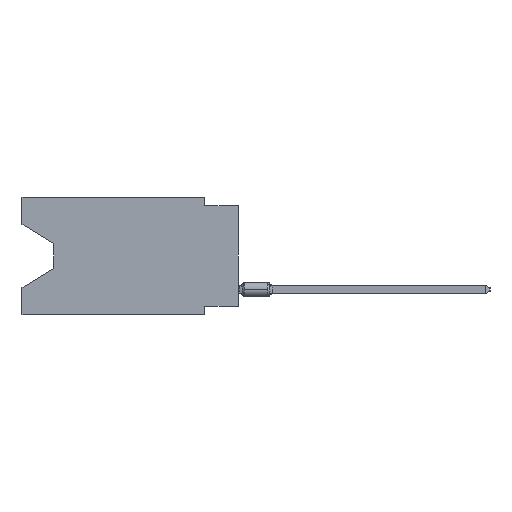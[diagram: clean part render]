
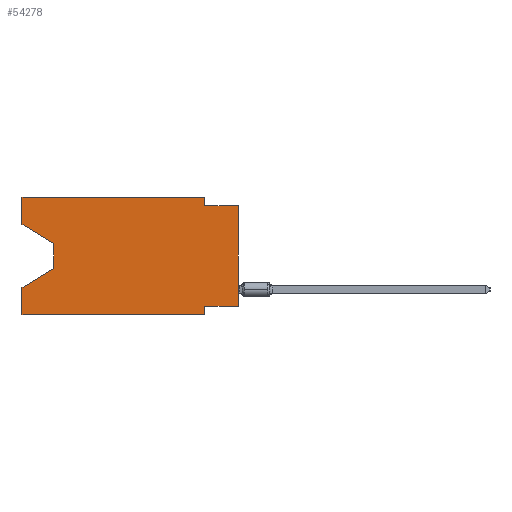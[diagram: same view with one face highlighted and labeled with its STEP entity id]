
A CAD part, left-side view. The second image highlights one B-rep face of the part: STEP entity #54278.
In plain terms, the highlighted planar face has unit normal (-1, 0, 0).
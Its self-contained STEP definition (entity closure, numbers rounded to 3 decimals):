
#98 = VERTEX_POINT ( 'NONE', #68388 ) ;
#173 = CARTESIAN_POINT ( 'NONE',  ( 0., 16.383, -2.038 ) ) ;
#647 = LINE ( 'NONE', #6383, #62513 ) ;
#803 = VERTEX_POINT ( 'NONE', #11691 ) ;
#1024 = CARTESIAN_POINT ( 'NONE',  ( 0., 2.54, 0. ) ) ;
#2046 = CARTESIAN_POINT ( 'NONE',  ( 0., 0., -0.635 ) ) ;
#2863 = CARTESIAN_POINT ( 'NONE',  ( 0., 0., -8.255 ) ) ;
#4618 = VECTOR ( 'NONE', #35750, 1000. ) ;
#4832 = ORIENTED_EDGE ( 'NONE', *, *, #60433, .F. ) ;
#4844 = DIRECTION ( 'NONE',  ( 1., 0., 0. ) ) ;
#5903 = ORIENTED_EDGE ( 'NONE', *, *, #38553, .F. ) ;
#6383 = CARTESIAN_POINT ( 'NONE',  ( 0., 2.54, -8.89 ) ) ;
#6622 = VERTEX_POINT ( 'NONE', #2046 ) ;
#7238 = VERTEX_POINT ( 'NONE', #21267 ) ;
#7702 = VERTEX_POINT ( 'NONE', #26556 ) ;
#7793 = LINE ( 'NONE', #13882, #4618 ) ;
#10424 = DIRECTION ( 'NONE',  ( 0., 0., -1. ) ) ;
#10850 = VECTOR ( 'NONE', #50318, 1000. ) ;
#11691 = CARTESIAN_POINT ( 'NONE',  ( 0., 16.383, -6.852 ) ) ;
#11999 = VERTEX_POINT ( 'NONE', #21408 ) ;
#12059 = VERTEX_POINT ( 'NONE', #63970 ) ;
#12400 = VECTOR ( 'NONE', #52069, 1000. ) ;
#12477 = LINE ( 'NONE', #60196, #29740 ) ;
#13882 = CARTESIAN_POINT ( 'NONE',  ( 0., 16.383, -8.89 ) ) ;
#14146 = DIRECTION ( 'NONE',  ( 0., -1., 0. ) ) ;
#14391 = ORIENTED_EDGE ( 'NONE', *, *, #19158, .T. ) ;
#15102 = LINE ( 'NONE', #49495, #58125 ) ;
#16674 = LINE ( 'NONE', #17024, #32114 ) ;
#16885 = ORIENTED_EDGE ( 'NONE', *, *, #63911, .T. ) ;
#16902 = ORIENTED_EDGE ( 'NONE', *, *, #58540, .F. ) ;
#16989 = DIRECTION ( 'NONE',  ( 0., -0.855, -0.519 ) ) ;
#17024 = CARTESIAN_POINT ( 'NONE',  ( 0., 16.383, 0. ) ) ;
#17244 = VECTOR ( 'NONE', #65752, 1000. ) ;
#18038 = LINE ( 'NONE', #61786, #10850 ) ;
#19158 = EDGE_CURVE ( 'NONE', #61972, #803, #39557, .T. ) ;
#19349 = CARTESIAN_POINT ( 'NONE',  ( 0., 13.97, -5.385 ) ) ;
#19780 = CARTESIAN_POINT ( 'NONE',  ( 0., 16.383, -2.038 ) ) ;
#19955 = EDGE_CURVE ( 'NONE', #28288, #98, #7793, .T. ) ;
#21267 = CARTESIAN_POINT ( 'NONE',  ( 0., 0., -8.255 ) ) ;
#21408 = CARTESIAN_POINT ( 'NONE',  ( 0., 2.54, -8.255 ) ) ;
#24356 = LINE ( 'NONE', #2863, #69401 ) ;
#24886 = CARTESIAN_POINT ( 'NONE',  ( 0., 0., -0.635 ) ) ;
#25729 = ORIENTED_EDGE ( 'NONE', *, *, #46327, .F. ) ;
#26556 = CARTESIAN_POINT ( 'NONE',  ( 0., 16.383, 0. ) ) ;
#27770 = LINE ( 'NONE', #173, #58589 ) ;
#28202 = EDGE_CURVE ( 'NONE', #7702, #62309, #16674, .T. ) ;
#28288 = VERTEX_POINT ( 'NONE', #50019 ) ;
#29740 = VECTOR ( 'NONE', #55179, 1000. ) ;
#31067 = CARTESIAN_POINT ( 'NONE',  ( 0., 0., 0. ) ) ;
#31907 = ORIENTED_EDGE ( 'NONE', *, *, #28202, .F. ) ;
#32114 = VECTOR ( 'NONE', #50374, 1000. ) ;
#33400 = VERTEX_POINT ( 'NONE', #19780 ) ;
#35750 = DIRECTION ( 'NONE',  ( 0., -1., 0. ) ) ;
#36972 = ORIENTED_EDGE ( 'NONE', *, *, #19955, .T. ) ;
#37052 = ORIENTED_EDGE ( 'NONE', *, *, #53569, .T. ) ;
#38553 = EDGE_CURVE ( 'NONE', #11999, #98, #647, .T. ) ;
#39366 = VECTOR ( 'NONE', #52949, 1000. ) ;
#39557 = LINE ( 'NONE', #45304, #17244 ) ;
#40271 = EDGE_LOOP ( 'NONE', ( #16885, #37052, #14391, #4832, #36972, #5903, #52904, #67574, #25729, #50634, #31907, #16902 ) ) ;
#40587 = VECTOR ( 'NONE', #14146, 1000. ) ;
#41610 = VERTEX_POINT ( 'NONE', #50727 ) ;
#44367 = DIRECTION ( 'NONE',  ( 0., 0., -1. ) ) ;
#45304 = CARTESIAN_POINT ( 'NONE',  ( 0., 13.97, -5.385 ) ) ;
#45912 = EDGE_CURVE ( 'NONE', #7238, #6622, #57978, .T. ) ;
#46327 = EDGE_CURVE ( 'NONE', #41610, #6622, #58243, .T. ) ;
#47180 = PLANE ( 'NONE',  #48131 ) ;
#47420 = CARTESIAN_POINT ( 'NONE',  ( 0., 16.383, 0. ) ) ;
#48131 = AXIS2_PLACEMENT_3D ( 'NONE', #53958, #4844, #69378 ) ;
#49495 = CARTESIAN_POINT ( 'NONE',  ( 0., 2.54, 0. ) ) ;
#50019 = CARTESIAN_POINT ( 'NONE',  ( 0., 16.383, -8.89 ) ) ;
#50318 = DIRECTION ( 'NONE',  ( 0., 0., 1. ) ) ;
#50374 = DIRECTION ( 'NONE',  ( 0., -1., 0. ) ) ;
#50634 = ORIENTED_EDGE ( 'NONE', *, *, #50919, .F. ) ;
#50727 = CARTESIAN_POINT ( 'NONE',  ( 0., 2.54, -0.635 ) ) ;
#50919 = EDGE_CURVE ( 'NONE', #62309, #41610, #15102, .T. ) ;
#52069 = DIRECTION ( 'NONE',  ( 0., 0., 1. ) ) ;
#52546 = FACE_OUTER_BOUND ( 'NONE', #40271, .T. ) ;
#52904 = ORIENTED_EDGE ( 'NONE', *, *, #59123, .F. ) ;
#52949 = DIRECTION ( 'NONE',  ( 0., 0., 1. ) ) ;
#53569 = EDGE_CURVE ( 'NONE', #12059, #61972, #12477, .T. ) ;
#53958 = CARTESIAN_POINT ( 'NONE',  ( 0., 16.383, 0. ) ) ;
#54278 = ADVANCED_FACE ( 'NONE', ( #52546 ), #47180, .F. ) ;
#55179 = DIRECTION ( 'NONE',  ( 0., 0., -1. ) ) ;
#57458 = LINE ( 'NONE', #47420, #12400 ) ;
#57978 = LINE ( 'NONE', #31067, #39366 ) ;
#58125 = VECTOR ( 'NONE', #10424, 1000. ) ;
#58243 = LINE ( 'NONE', #24886, #40587 ) ;
#58540 = EDGE_CURVE ( 'NONE', #33400, #7702, #18038, .T. ) ;
#58589 = VECTOR ( 'NONE', #16989, 1000. ) ;
#59123 = EDGE_CURVE ( 'NONE', #7238, #11999, #24356, .T. ) ;
#60196 = CARTESIAN_POINT ( 'NONE',  ( 0., 13.97, -3.505 ) ) ;
#60433 = EDGE_CURVE ( 'NONE', #28288, #803, #57458, .T. ) ;
#61786 = CARTESIAN_POINT ( 'NONE',  ( 0., 16.383, 0. ) ) ;
#61972 = VERTEX_POINT ( 'NONE', #19349 ) ;
#62309 = VERTEX_POINT ( 'NONE', #1024 ) ;
#62513 = VECTOR ( 'NONE', #44367, 1000. ) ;
#62729 = DIRECTION ( 'NONE',  ( 0., 1., 0. ) ) ;
#63911 = EDGE_CURVE ( 'NONE', #33400, #12059, #27770, .T. ) ;
#63970 = CARTESIAN_POINT ( 'NONE',  ( 0., 13.97, -3.505 ) ) ;
#65752 = DIRECTION ( 'NONE',  ( 0., 0.855, -0.519 ) ) ;
#67574 = ORIENTED_EDGE ( 'NONE', *, *, #45912, .T. ) ;
#68388 = CARTESIAN_POINT ( 'NONE',  ( 0., 2.54, -8.89 ) ) ;
#69378 = DIRECTION ( 'NONE',  ( 0., 0., -1. ) ) ;
#69401 = VECTOR ( 'NONE', #62729, 1000. ) ;
